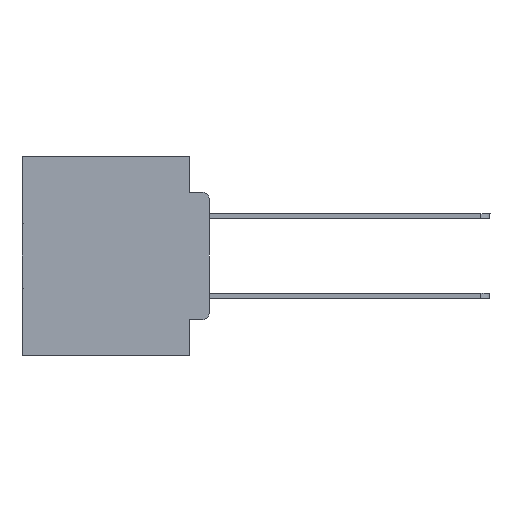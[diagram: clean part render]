
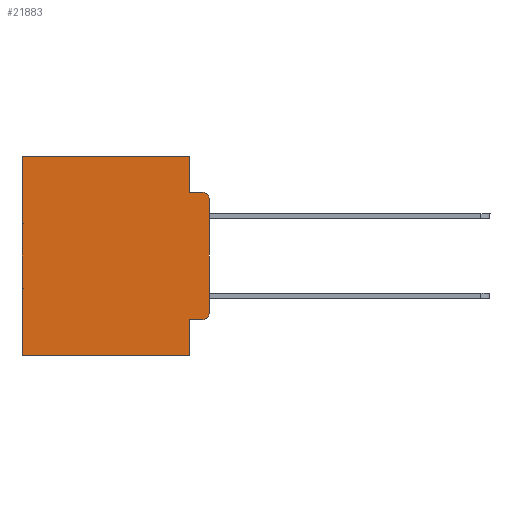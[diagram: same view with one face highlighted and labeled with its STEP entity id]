
A CAD part, left-side view. The second image highlights one B-rep face of the part: STEP entity #21883.
In plain terms, the highlighted planar face has unit normal (-1, 0, 0).
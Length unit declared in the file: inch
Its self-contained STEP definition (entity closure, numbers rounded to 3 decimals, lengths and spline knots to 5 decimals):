
#116 = LINE ( 'NONE', #31080, #32196 ) ;
#480 = VERTEX_POINT ( 'NONE', #7521 ) ;
#516 = ORIENTED_EDGE ( 'NONE', *, *, #12653, .T. ) ;
#898 = ORIENTED_EDGE ( 'NONE', *, *, #32931, .T. ) ;
#1743 = CARTESIAN_POINT ( 'NONE',  ( 0.298, 0.051, 0. ) ) ;
#1775 = CARTESIAN_POINT ( 'NONE',  ( 0.298, 0.02, -0.3915 ) ) ;
#1832 = CARTESIAN_POINT ( 'NONE',  ( 0.298, 0., -0.5 ) ) ;
#1990 = DIRECTION ( 'NONE',  ( 0., -1., 0. ) ) ;
#1997 = CARTESIAN_POINT ( 'NONE',  ( 0.298, 0.051, -0.5 ) ) ;
#2039 = AXIS2_PLACEMENT_3D ( 'NONE', #1775, #11731, #12065 ) ;
#2083 = DIRECTION ( 'NONE',  ( 0., 0., -1. ) ) ;
#2297 = LINE ( 'NONE', #9739, #29885 ) ;
#2678 = AXIS2_PLACEMENT_3D ( 'NONE', #29805, #4567, #27970 ) ;
#3220 = ORIENTED_EDGE ( 'NONE', *, *, #15519, .F. ) ;
#3646 = DIRECTION ( 'NONE',  ( 0., 0., -1. ) ) ;
#3906 = VERTEX_POINT ( 'NONE', #25563 ) ;
#4288 = VECTOR ( 'NONE', #3646, 39.37008 ) ;
#4567 = DIRECTION ( 'NONE',  ( -1., 0., 0. ) ) ;
#5220 = CARTESIAN_POINT ( 'NONE',  ( 0.298, 0., -0.1085 ) ) ;
#5816 = CARTESIAN_POINT ( 'NONE',  ( 0.298, 0.473, -0.5 ) ) ;
#6136 = AXIS2_PLACEMENT_3D ( 'NONE', #11537, #32191, #29675 ) ;
#6190 = LINE ( 'NONE', #26713, #4288 ) ;
#6449 = VECTOR ( 'NONE', #29480, 39.37008 ) ;
#7007 = VERTEX_POINT ( 'NONE', #5220 ) ;
#7212 = CARTESIAN_POINT ( 'NONE',  ( 0.298, 0.051, -0.0885 ) ) ;
#7371 = EDGE_CURVE ( 'NONE', #28675, #23064, #16665, .T. ) ;
#7521 = CARTESIAN_POINT ( 'NONE',  ( 0.298, 0., -0.3915 ) ) ;
#8101 = VERTEX_POINT ( 'NONE', #16058 ) ;
#9125 = LINE ( 'NONE', #13872, #6449 ) ;
#9660 = VECTOR ( 'NONE', #24808, 39.37008 ) ;
#9739 = CARTESIAN_POINT ( 'NONE',  ( 0.298, 0.051, -0.4115 ) ) ;
#11016 = EDGE_CURVE ( 'NONE', #31295, #24157, #2297, .T. ) ;
#11288 = CARTESIAN_POINT ( 'NONE',  ( 0.298, 0.02, -0.4115 ) ) ;
#11537 = CARTESIAN_POINT ( 'NONE',  ( 0.298, 0., 0. ) ) ;
#11731 = DIRECTION ( 'NONE',  ( -1., 0., 0. ) ) ;
#12065 = DIRECTION ( 'NONE',  ( 0., 0., -1. ) ) ;
#12587 = DIRECTION ( 'NONE',  ( 0., -1., 0. ) ) ;
#12653 = EDGE_CURVE ( 'NONE', #24157, #480, #16558, .T. ) ;
#13034 = ORIENTED_EDGE ( 'NONE', *, *, #15503, .T. ) ;
#13254 = VERTEX_POINT ( 'NONE', #24063 ) ;
#13872 = CARTESIAN_POINT ( 'NONE',  ( 0.298, 0., 0. ) ) ;
#14320 = DIRECTION ( 'NONE',  ( 0., 1., 0. ) ) ;
#15503 = EDGE_CURVE ( 'NONE', #13254, #8101, #116, .T. ) ;
#15519 = EDGE_CURVE ( 'NONE', #31295, #28675, #21805, .T. ) ;
#15958 = EDGE_CURVE ( 'NONE', #7007, #480, #9125, .T. ) ;
#16058 = CARTESIAN_POINT ( 'NONE',  ( 0.298, 0.473, 0. ) ) ;
#16081 = EDGE_CURVE ( 'NONE', #7007, #21534, #24172, .T. ) ;
#16558 = CIRCLE ( 'NONE', #2039, 0.02 ) ;
#16665 = LINE ( 'NONE', #1832, #26963 ) ;
#17443 = ORIENTED_EDGE ( 'NONE', *, *, #7371, .F. ) ;
#17451 = VECTOR ( 'NONE', #2083, 39.37008 ) ;
#19297 = CARTESIAN_POINT ( 'NONE',  ( 0.298, 0.051, 0. ) ) ;
#21300 = VECTOR ( 'NONE', #1990, 39.37008 ) ;
#21534 = VERTEX_POINT ( 'NONE', #27836 ) ;
#21538 = EDGE_CURVE ( 'NONE', #13254, #3906, #30504, .T. ) ;
#21805 = LINE ( 'NONE', #19297, #9660 ) ;
#21883 = ADVANCED_FACE ( 'NONE', ( #21969 ), #24138, .F. ) ;
#21969 = FACE_OUTER_BOUND ( 'NONE', #23881, .T. ) ;
#22029 = LINE ( 'NONE', #7212, #21300 ) ;
#22377 = CARTESIAN_POINT ( 'NONE',  ( 0.298, 0.051, -0.4115 ) ) ;
#23064 = VERTEX_POINT ( 'NONE', #5816 ) ;
#23881 = EDGE_LOOP ( 'NONE', ( #29492, #24416, #25926, #31371, #13034, #898, #17443, #3220, #29455, #516 ) ) ;
#24063 = CARTESIAN_POINT ( 'NONE',  ( 0.298, 0.051, 0. ) ) ;
#24138 = PLANE ( 'NONE',  #6136 ) ;
#24157 = VERTEX_POINT ( 'NONE', #11288 ) ;
#24172 = CIRCLE ( 'NONE', #2678, 0.02 ) ;
#24416 = ORIENTED_EDGE ( 'NONE', *, *, #16081, .T. ) ;
#24808 = DIRECTION ( 'NONE',  ( 0., 0., -1. ) ) ;
#25563 = CARTESIAN_POINT ( 'NONE',  ( 0.298, 0.051, -0.0885 ) ) ;
#25926 = ORIENTED_EDGE ( 'NONE', *, *, #27471, .F. ) ;
#26713 = CARTESIAN_POINT ( 'NONE',  ( 0.298, 0.473, 0. ) ) ;
#26963 = VECTOR ( 'NONE', #14320, 39.37008 ) ;
#27471 = EDGE_CURVE ( 'NONE', #3906, #21534, #22029, .T. ) ;
#27836 = CARTESIAN_POINT ( 'NONE',  ( 0.298, 0.02, -0.0885 ) ) ;
#27970 = DIRECTION ( 'NONE',  ( 0., 0., -1. ) ) ;
#28675 = VERTEX_POINT ( 'NONE', #1997 ) ;
#29356 = DIRECTION ( 'NONE',  ( 0., 1., 0. ) ) ;
#29455 = ORIENTED_EDGE ( 'NONE', *, *, #11016, .T. ) ;
#29480 = DIRECTION ( 'NONE',  ( 0., 0., -1. ) ) ;
#29492 = ORIENTED_EDGE ( 'NONE', *, *, #15958, .F. ) ;
#29675 = DIRECTION ( 'NONE',  ( 0., 0., -1. ) ) ;
#29805 = CARTESIAN_POINT ( 'NONE',  ( 0.298, 0.02, -0.1085 ) ) ;
#29885 = VECTOR ( 'NONE', #12587, 39.37008 ) ;
#30504 = LINE ( 'NONE', #1743, #17451 ) ;
#31080 = CARTESIAN_POINT ( 'NONE',  ( 0.298, 0., 0. ) ) ;
#31295 = VERTEX_POINT ( 'NONE', #22377 ) ;
#31371 = ORIENTED_EDGE ( 'NONE', *, *, #21538, .F. ) ;
#32191 = DIRECTION ( 'NONE',  ( 1., 0., 0. ) ) ;
#32196 = VECTOR ( 'NONE', #29356, 39.37008 ) ;
#32931 = EDGE_CURVE ( 'NONE', #8101, #23064, #6190, .T. ) ;
